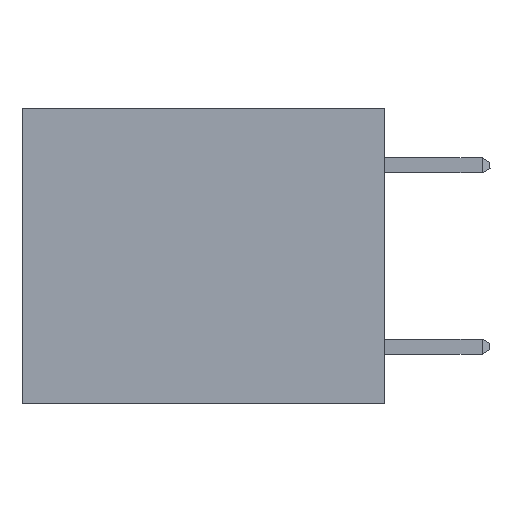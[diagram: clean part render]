
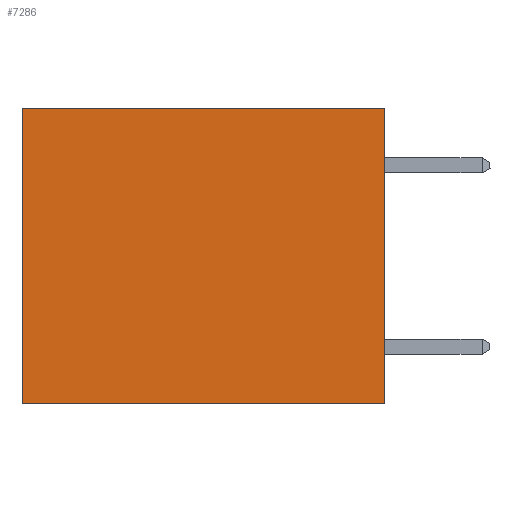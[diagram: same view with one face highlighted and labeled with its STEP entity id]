
A CAD part, left-side view. The second image highlights one B-rep face of the part: STEP entity #7286.
In plain terms, the highlighted planar face has unit normal (-1, 0, 0).
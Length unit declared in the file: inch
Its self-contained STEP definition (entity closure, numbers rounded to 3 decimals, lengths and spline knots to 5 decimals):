
#9 = LINE ( 'NONE', #1714, #27613 ) ;
#171 = ORIENTED_EDGE ( 'NONE', *, *, #15886, .T. ) ;
#1714 = CARTESIAN_POINT ( 'NONE',  ( 0.3165, 0., 0. ) ) ;
#3720 = CARTESIAN_POINT ( 'NONE',  ( 0.3165, 0., -0.49 ) ) ;
#3826 = VECTOR ( 'NONE', #23956, 39.37008 ) ;
#3838 = VERTEX_POINT ( 'NONE', #17158 ) ;
#4176 = LINE ( 'NONE', #18644, #3826 ) ;
#5456 = EDGE_CURVE ( 'NONE', #19270, #29154, #9, .T. ) ;
#5595 = LINE ( 'NONE', #20943, #28689 ) ;
#5796 = CARTESIAN_POINT ( 'NONE',  ( 0.3165, 0., -0.49 ) ) ;
#7286 = ADVANCED_FACE ( 'NONE', ( #12393 ), #15659, .F. ) ;
#8142 = DIRECTION ( 'NONE',  ( 0., 0., -1. ) ) ;
#8716 = EDGE_CURVE ( 'NONE', #19270, #12646, #13800, .T. ) ;
#9563 = EDGE_CURVE ( 'NONE', #12646, #3838, #5595, .T. ) ;
#10432 = DIRECTION ( 'NONE',  ( 0., 1., 0. ) ) ;
#11083 = DIRECTION ( 'NONE',  ( 0., 1., 0. ) ) ;
#12393 = FACE_OUTER_BOUND ( 'NONE', #21067, .T. ) ;
#12646 = VERTEX_POINT ( 'NONE', #3720 ) ;
#13800 = LINE ( 'NONE', #25452, #28742 ) ;
#15659 = PLANE ( 'NONE',  #22764 ) ;
#15886 = EDGE_CURVE ( 'NONE', #29154, #3838, #4176, .T. ) ;
#17158 = CARTESIAN_POINT ( 'NONE',  ( 0.3165, 0.6, -0.49 ) ) ;
#18644 = CARTESIAN_POINT ( 'NONE',  ( 0.3165, 0.6, -0.49 ) ) ;
#19270 = VERTEX_POINT ( 'NONE', #22403 ) ;
#20720 = ORIENTED_EDGE ( 'NONE', *, *, #5456, .T. ) ;
#20943 = CARTESIAN_POINT ( 'NONE',  ( 0.3165, 0., -0.49 ) ) ;
#21067 = EDGE_LOOP ( 'NONE', ( #171, #22720, #27813, #20720 ) ) ;
#22393 = DIRECTION ( 'NONE',  ( 1., 0., 0. ) ) ;
#22403 = CARTESIAN_POINT ( 'NONE',  ( 0.3165, 0., 0. ) ) ;
#22720 = ORIENTED_EDGE ( 'NONE', *, *, #9563, .F. ) ;
#22764 = AXIS2_PLACEMENT_3D ( 'NONE', #5796, #22393, #8142 ) ;
#23956 = DIRECTION ( 'NONE',  ( 0., 0., -1. ) ) ;
#25452 = CARTESIAN_POINT ( 'NONE',  ( 0.3165, 0., -0.49 ) ) ;
#25892 = CARTESIAN_POINT ( 'NONE',  ( 0.3165, 0.6, 0. ) ) ;
#27613 = VECTOR ( 'NONE', #10432, 39.37008 ) ;
#27813 = ORIENTED_EDGE ( 'NONE', *, *, #8716, .F. ) ;
#28689 = VECTOR ( 'NONE', #11083, 39.37008 ) ;
#28742 = VECTOR ( 'NONE', #30566, 39.37008 ) ;
#29154 = VERTEX_POINT ( 'NONE', #25892 ) ;
#30566 = DIRECTION ( 'NONE',  ( 0., 0., -1. ) ) ;
